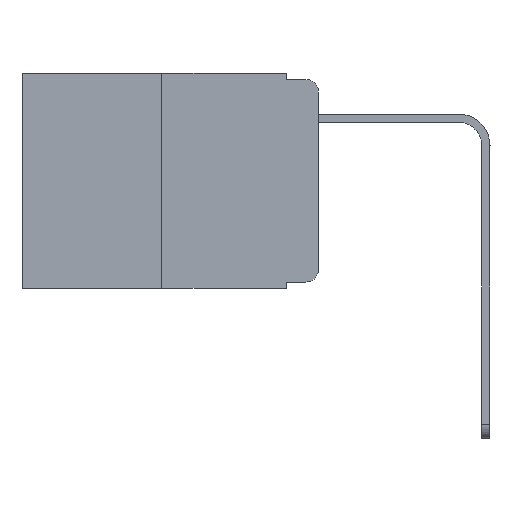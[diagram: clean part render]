
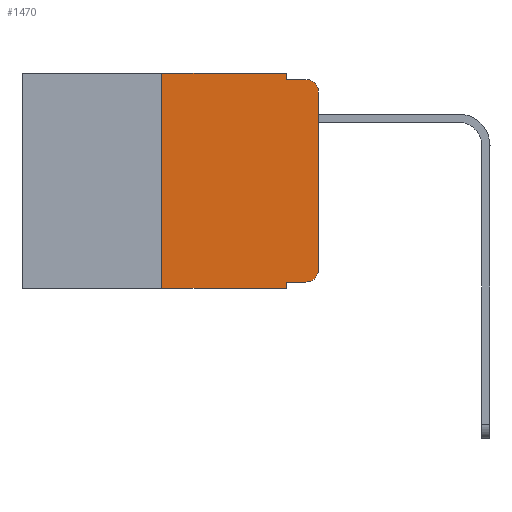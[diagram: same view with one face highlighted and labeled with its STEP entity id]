
A CAD part, left-side view. The second image highlights one B-rep face of the part: STEP entity #1470.
In plain terms, the highlighted planar face has unit normal (-1, 0, 0).
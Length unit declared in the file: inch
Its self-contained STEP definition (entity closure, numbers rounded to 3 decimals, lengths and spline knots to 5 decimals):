
#93 = DIRECTION ( 'NONE',  ( -1., 0., 0. ) ) ;
#338 = PLANE ( 'NONE',  #6806 ) ;
#418 = ORIENTED_EDGE ( 'NONE', *, *, #1164, .F. ) ;
#496 = CARTESIAN_POINT ( 'NONE',  ( 0., 0.25, 0. ) ) ;
#769 = CARTESIAN_POINT ( 'NONE',  ( 0., 0.051, 0. ) ) ;
#1164 = EDGE_CURVE ( 'NONE', #12165, #2963, #5291, .T. ) ;
#1250 = VECTOR ( 'NONE', #5947, 39.37008 ) ;
#1281 = DIRECTION ( 'NONE',  ( 0., 0., -1. ) ) ;
#1421 = CARTESIAN_POINT ( 'NONE',  ( 0., 0.02, -0.333 ) ) ;
#1446 = VERTEX_POINT ( 'NONE', #1421 ) ;
#1470 = ADVANCED_FACE ( 'NONE', ( #4397 ), #338, .F. ) ;
#1527 = EDGE_CURVE ( 'NONE', #12165, #1446, #9881, .T. ) ;
#1881 = CARTESIAN_POINT ( 'NONE',  ( 0., 0.473, 0. ) ) ;
#2147 = VECTOR ( 'NONE', #6867, 39.37008 ) ;
#2694 = LINE ( 'NONE', #7613, #10232 ) ;
#2717 = CIRCLE ( 'NONE', #4546, 0.02 ) ;
#2963 = VERTEX_POINT ( 'NONE', #6668 ) ;
#3217 = VECTOR ( 'NONE', #9094, 39.37008 ) ;
#3332 = CARTESIAN_POINT ( 'NONE',  ( 0., 0.051, -0.01 ) ) ;
#3380 = VERTEX_POINT ( 'NONE', #3701 ) ;
#3398 = VECTOR ( 'NONE', #5426, 39.37008 ) ;
#3467 = CARTESIAN_POINT ( 'NONE',  ( 0., 0., 0. ) ) ;
#3541 = CARTESIAN_POINT ( 'NONE',  ( 0., 0.051, -0.333 ) ) ;
#3626 = VERTEX_POINT ( 'NONE', #8846 ) ;
#3701 = CARTESIAN_POINT ( 'NONE',  ( 0., 0.051, 0. ) ) ;
#3763 = CARTESIAN_POINT ( 'NONE',  ( 0., 0.051, -0.333 ) ) ;
#4131 = EDGE_CURVE ( 'NONE', #4773, #2963, #2694, .T. ) ;
#4238 = DIRECTION ( 'NONE',  ( -1., 0., 0. ) ) ;
#4397 = FACE_OUTER_BOUND ( 'NONE', #11623, .T. ) ;
#4533 = CARTESIAN_POINT ( 'NONE',  ( 0., 0.02, -0.03 ) ) ;
#4546 = AXIS2_PLACEMENT_3D ( 'NONE', #11929, #4238, #5354 ) ;
#4735 = DIRECTION ( 'NONE',  ( 0., 0., -1. ) ) ;
#4746 = DIRECTION ( 'NONE',  ( 0., 0., 1. ) ) ;
#4773 = VERTEX_POINT ( 'NONE', #11080 ) ;
#5291 = LINE ( 'NONE', #8454, #3398 ) ;
#5354 = DIRECTION ( 'NONE',  ( 0., 0., -1. ) ) ;
#5426 = DIRECTION ( 'NONE',  ( 0., 0., -1. ) ) ;
#5509 = EDGE_CURVE ( 'NONE', #9080, #8129, #10528, .T. ) ;
#5547 = ORIENTED_EDGE ( 'NONE', *, *, #11844, .T. ) ;
#5548 = VECTOR ( 'NONE', #5809, 39.37008 ) ;
#5809 = DIRECTION ( 'NONE',  ( 0., 0., 1. ) ) ;
#5871 = LINE ( 'NONE', #1881, #9130 ) ;
#5940 = ORIENTED_EDGE ( 'NONE', *, *, #11437, .F. ) ;
#5947 = DIRECTION ( 'NONE',  ( 0., 0., -1. ) ) ;
#6269 = CARTESIAN_POINT ( 'NONE',  ( 0., 0., -0.03 ) ) ;
#6384 = EDGE_CURVE ( 'NONE', #1446, #9080, #2717, .T. ) ;
#6668 = CARTESIAN_POINT ( 'NONE',  ( 0., 0.051, -0.343 ) ) ;
#6806 = AXIS2_PLACEMENT_3D ( 'NONE', #11224, #7889, #4735 ) ;
#6867 = DIRECTION ( 'NONE',  ( 0., -1., 0. ) ) ;
#7094 = ORIENTED_EDGE ( 'NONE', *, *, #1527, .T. ) ;
#7438 = AXIS2_PLACEMENT_3D ( 'NONE', #4533, #93, #1281 ) ;
#7613 = CARTESIAN_POINT ( 'NONE',  ( 0., 0.473, -0.343 ) ) ;
#7671 = EDGE_CURVE ( 'NONE', #8904, #10175, #11063, .T. ) ;
#7889 = DIRECTION ( 'NONE',  ( 1., 0., 0. ) ) ;
#7898 = ORIENTED_EDGE ( 'NONE', *, *, #12666, .F. ) ;
#8129 = VERTEX_POINT ( 'NONE', #6269 ) ;
#8440 = VECTOR ( 'NONE', #4746, 39.37008 ) ;
#8454 = CARTESIAN_POINT ( 'NONE',  ( 0., 0.051, 0. ) ) ;
#8666 = ORIENTED_EDGE ( 'NONE', *, *, #6384, .T. ) ;
#8788 = CARTESIAN_POINT ( 'NONE',  ( 0., 0.02, -0.01 ) ) ;
#8846 = CARTESIAN_POINT ( 'NONE',  ( 0., 0.25, 0. ) ) ;
#8904 = VERTEX_POINT ( 'NONE', #9064 ) ;
#9064 = CARTESIAN_POINT ( 'NONE',  ( 0., 0.051, -0.01 ) ) ;
#9080 = VERTEX_POINT ( 'NONE', #10593 ) ;
#9094 = DIRECTION ( 'NONE',  ( 0., -1., 0. ) ) ;
#9130 = VECTOR ( 'NONE', #10481, 39.37008 ) ;
#9342 = ORIENTED_EDGE ( 'NONE', *, *, #11560, .F. ) ;
#9388 = ORIENTED_EDGE ( 'NONE', *, *, #4131, .T. ) ;
#9881 = LINE ( 'NONE', #3541, #3217 ) ;
#9955 = DIRECTION ( 'NONE',  ( 0., -1., 0. ) ) ;
#10175 = VERTEX_POINT ( 'NONE', #8788 ) ;
#10232 = VECTOR ( 'NONE', #9955, 39.37008 ) ;
#10481 = DIRECTION ( 'NONE',  ( 0., -1., 0. ) ) ;
#10528 = LINE ( 'NONE', #3467, #5548 ) ;
#10593 = CARTESIAN_POINT ( 'NONE',  ( 0., 0., -0.313 ) ) ;
#10819 = LINE ( 'NONE', #769, #1250 ) ;
#10930 = ORIENTED_EDGE ( 'NONE', *, *, #7671, .F. ) ;
#11063 = LINE ( 'NONE', #3332, #2147 ) ;
#11080 = CARTESIAN_POINT ( 'NONE',  ( 0., 0.25, -0.343 ) ) ;
#11224 = CARTESIAN_POINT ( 'NONE',  ( 0., 0.473, 0. ) ) ;
#11437 = EDGE_CURVE ( 'NONE', #4773, #3626, #13736, .T. ) ;
#11560 = EDGE_CURVE ( 'NONE', #3626, #3380, #5871, .T. ) ;
#11623 = EDGE_LOOP ( 'NONE', ( #13670, #5547, #10930, #7898, #9342, #5940, #9388, #418, #7094, #8666 ) ) ;
#11844 = EDGE_CURVE ( 'NONE', #8129, #10175, #12365, .T. ) ;
#11929 = CARTESIAN_POINT ( 'NONE',  ( 0., 0.02, -0.313 ) ) ;
#12165 = VERTEX_POINT ( 'NONE', #3763 ) ;
#12365 = CIRCLE ( 'NONE', #7438, 0.02 ) ;
#12666 = EDGE_CURVE ( 'NONE', #3380, #8904, #10819, .T. ) ;
#13670 = ORIENTED_EDGE ( 'NONE', *, *, #5509, .T. ) ;
#13736 = LINE ( 'NONE', #496, #8440 ) ;
